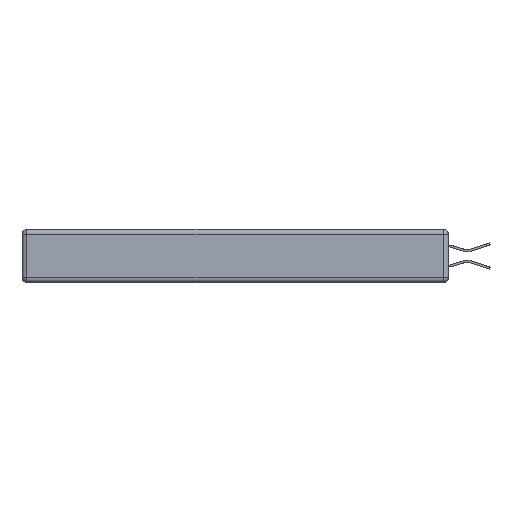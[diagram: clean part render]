
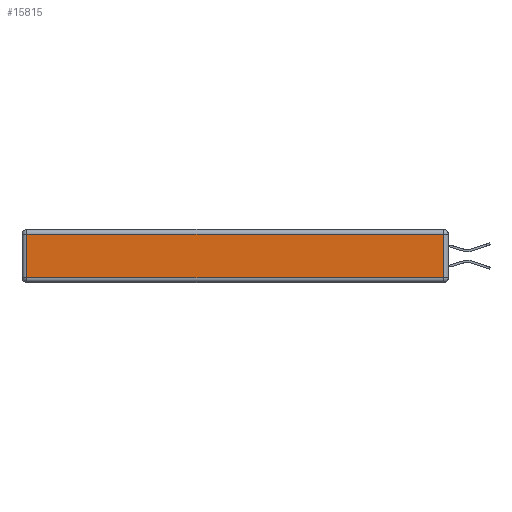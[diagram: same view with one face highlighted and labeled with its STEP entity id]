
A CAD part, left-side view. The second image highlights one B-rep face of the part: STEP entity #15815.
In plain terms, the highlighted planar face has unit normal (-1, 0, 0).
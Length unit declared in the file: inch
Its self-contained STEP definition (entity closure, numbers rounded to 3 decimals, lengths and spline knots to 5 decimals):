
#390 = CARTESIAN_POINT ( 'NONE',  ( 0., 0.03, -0.343 ) ) ;
#831 = VERTEX_POINT ( 'NONE', #20533 ) ;
#1547 = DIRECTION ( 'NONE',  ( -1., 0., 0. ) ) ;
#1823 = CARTESIAN_POINT ( 'NONE',  ( 0., 0.03, -0.03 ) ) ;
#2182 = ORIENTED_EDGE ( 'NONE', *, *, #16888, .T. ) ;
#2336 = CARTESIAN_POINT ( 'NONE',  ( 0., 0.03, -0.313 ) ) ;
#2566 = ORIENTED_EDGE ( 'NONE', *, *, #19192, .T. ) ;
#3418 = LINE ( 'NONE', #15466, #18523 ) ;
#3468 = VERTEX_POINT ( 'NONE', #1823 ) ;
#4803 = EDGE_CURVE ( 'NONE', #19610, #3468, #11869, .T. ) ;
#6635 = FACE_OUTER_BOUND ( 'NONE', #12085, .T. ) ;
#6686 = DIRECTION ( 'NONE',  ( 0., 0., 1. ) ) ;
#7859 = ORIENTED_EDGE ( 'NONE', *, *, #4803, .T. ) ;
#10156 = DIRECTION ( 'NONE',  ( 0., 1., 0. ) ) ;
#11686 = PLANE ( 'NONE',  #12305 ) ;
#11869 = LINE ( 'NONE', #390, #14265 ) ;
#12085 = EDGE_LOOP ( 'NONE', ( #17802, #7859, #2182, #2566 ) ) ;
#12305 = AXIS2_PLACEMENT_3D ( 'NONE', #16851, #1547, #6686 ) ;
#12577 = VERTEX_POINT ( 'NONE', #13176 ) ;
#13176 = CARTESIAN_POINT ( 'NONE',  ( 0., 2.72, -0.03 ) ) ;
#14265 = VECTOR ( 'NONE', #20781, 39.37008 ) ;
#14347 = VECTOR ( 'NONE', #10156, 39.37008 ) ;
#15466 = CARTESIAN_POINT ( 'NONE',  ( 0., 2.72, -0.343 ) ) ;
#15815 = ADVANCED_FACE ( 'NONE', ( #6635 ), #11686, .T. ) ;
#16816 = VECTOR ( 'NONE', #19547, 39.37008 ) ;
#16851 = CARTESIAN_POINT ( 'NONE',  ( 0., 0., -0.343 ) ) ;
#16888 = EDGE_CURVE ( 'NONE', #3468, #12577, #20483, .T. ) ;
#17802 = ORIENTED_EDGE ( 'NONE', *, *, #20959, .T. ) ;
#18523 = VECTOR ( 'NONE', #18664, 39.37008 ) ;
#18664 = DIRECTION ( 'NONE',  ( 0., 0., -1. ) ) ;
#18960 = LINE ( 'NONE', #19393, #16816 ) ;
#19192 = EDGE_CURVE ( 'NONE', #12577, #831, #3418, .T. ) ;
#19393 = CARTESIAN_POINT ( 'NONE',  ( 0., 0., -0.313 ) ) ;
#19547 = DIRECTION ( 'NONE',  ( 0., -1., 0. ) ) ;
#19610 = VERTEX_POINT ( 'NONE', #2336 ) ;
#20251 = CARTESIAN_POINT ( 'NONE',  ( 0., 2.75, -0.03 ) ) ;
#20483 = LINE ( 'NONE', #20251, #14347 ) ;
#20533 = CARTESIAN_POINT ( 'NONE',  ( 0., 2.72, -0.313 ) ) ;
#20781 = DIRECTION ( 'NONE',  ( 0., 0., 1. ) ) ;
#20959 = EDGE_CURVE ( 'NONE', #831, #19610, #18960, .T. ) ;
